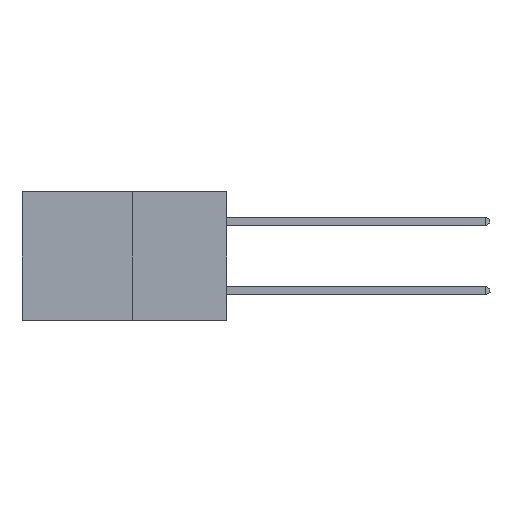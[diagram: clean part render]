
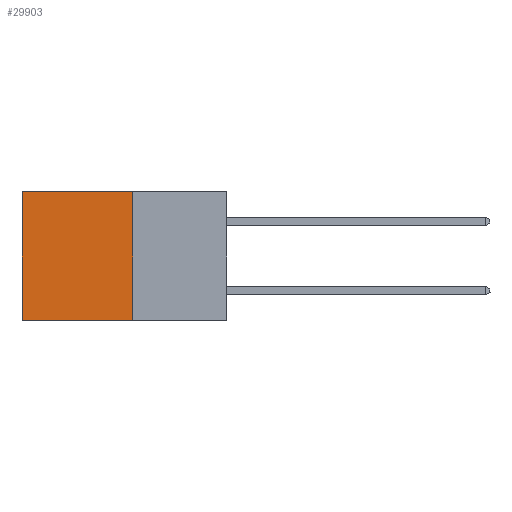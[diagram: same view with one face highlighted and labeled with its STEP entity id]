
A CAD part, left-side view. The second image highlights one B-rep face of the part: STEP entity #29903.
In plain terms, the highlighted planar face has unit normal (-1, 0, 0).
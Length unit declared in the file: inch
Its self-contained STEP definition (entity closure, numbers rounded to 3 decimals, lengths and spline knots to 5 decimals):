
#284 = LINE ( 'NONE', #16094, #20419 ) ;
#618 = CARTESIAN_POINT ( 'NONE',  ( 0.277, 0.59, 0. ) ) ;
#867 = FACE_OUTER_BOUND ( 'NONE', #29778, .T. ) ;
#1063 = ORIENTED_EDGE ( 'NONE', *, *, #26251, .F. ) ;
#3140 = PLANE ( 'NONE',  #23792 ) ;
#3328 = VERTEX_POINT ( 'NONE', #32963 ) ;
#4296 = CARTESIAN_POINT ( 'NONE',  ( 0.277, 0.27, -0.37 ) ) ;
#4848 = DIRECTION ( 'NONE',  ( 0., 1., 0. ) ) ;
#6663 = CARTESIAN_POINT ( 'NONE',  ( 0.277, 0.59, -0.37 ) ) ;
#6858 = VECTOR ( 'NONE', #4848, 39.37008 ) ;
#8371 = CARTESIAN_POINT ( 'NONE',  ( 0.277, 0.59, -0.37 ) ) ;
#9902 = ORIENTED_EDGE ( 'NONE', *, *, #25738, .F. ) ;
#10391 = CARTESIAN_POINT ( 'NONE',  ( 0.277, 0.27, 0. ) ) ;
#10532 = VECTOR ( 'NONE', #20863, 39.37008 ) ;
#10655 = VECTOR ( 'NONE', #11153, 39.37008 ) ;
#11153 = DIRECTION ( 'NONE',  ( 0., 0., -1. ) ) ;
#13504 = VERTEX_POINT ( 'NONE', #618 ) ;
#14077 = EDGE_CURVE ( 'NONE', #13504, #26848, #32394, .T. ) ;
#16094 = CARTESIAN_POINT ( 'NONE',  ( 0.277, 0.27, -0.37 ) ) ;
#16771 = ORIENTED_EDGE ( 'NONE', *, *, #14077, .T. ) ;
#16923 = DIRECTION ( 'NONE',  ( 0., 0., -1. ) ) ;
#18861 = DIRECTION ( 'NONE',  ( 0., 1., 0. ) ) ;
#20419 = VECTOR ( 'NONE', #18861, 39.37008 ) ;
#20863 = DIRECTION ( 'NONE',  ( 0., 0., -1. ) ) ;
#23792 = AXIS2_PLACEMENT_3D ( 'NONE', #30504, #33214, #16923 ) ;
#24118 = VERTEX_POINT ( 'NONE', #24560 ) ;
#24560 = CARTESIAN_POINT ( 'NONE',  ( 0.277, 0.27, -0.37 ) ) ;
#25738 = EDGE_CURVE ( 'NONE', #24118, #26848, #284, .T. ) ;
#26251 = EDGE_CURVE ( 'NONE', #3328, #24118, #33112, .T. ) ;
#26848 = VERTEX_POINT ( 'NONE', #6663 ) ;
#29016 = EDGE_CURVE ( 'NONE', #3328, #13504, #35017, .T. ) ;
#29751 = ORIENTED_EDGE ( 'NONE', *, *, #29016, .T. ) ;
#29778 = EDGE_LOOP ( 'NONE', ( #16771, #9902, #1063, #29751 ) ) ;
#29903 = ADVANCED_FACE ( 'NONE', ( #867 ), #3140, .F. ) ;
#30504 = CARTESIAN_POINT ( 'NONE',  ( 0.277, 0.27, -0.37 ) ) ;
#32394 = LINE ( 'NONE', #8371, #10655 ) ;
#32963 = CARTESIAN_POINT ( 'NONE',  ( 0.277, 0.27, 0. ) ) ;
#33112 = LINE ( 'NONE', #4296, #10532 ) ;
#33214 = DIRECTION ( 'NONE',  ( 1., 0., 0. ) ) ;
#35017 = LINE ( 'NONE', #10391, #6858 ) ;
